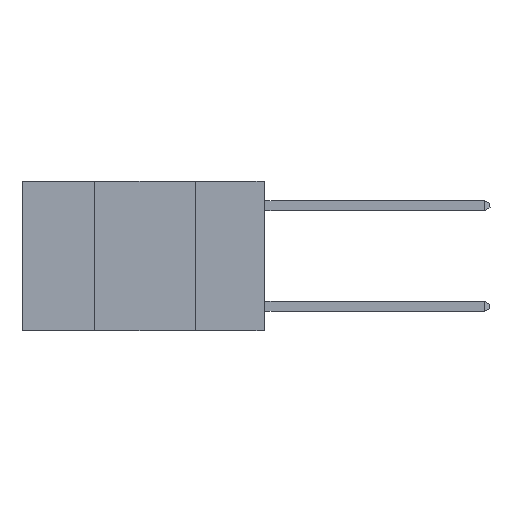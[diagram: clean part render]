
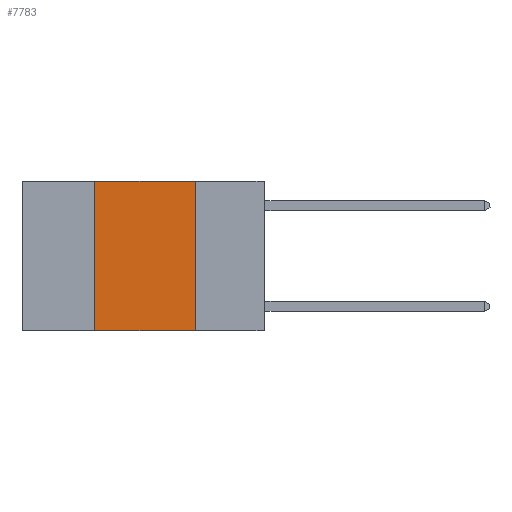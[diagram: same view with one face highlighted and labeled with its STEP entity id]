
A CAD part, left-side view. The second image highlights one B-rep face of the part: STEP entity #7783.
In plain terms, the highlighted planar face has unit normal (-1, 0, 0).
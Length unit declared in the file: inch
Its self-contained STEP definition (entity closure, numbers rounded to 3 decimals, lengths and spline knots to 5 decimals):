
#18 = CARTESIAN_POINT ( 'NONE',  ( 0., 0.6, 0. ) ) ;
#698 = DIRECTION ( 'NONE',  ( 0., -1., 0. ) ) ;
#1036 = PLANE ( 'NONE',  #8825 ) ;
#1455 = EDGE_CURVE ( 'NONE', #3841, #2883, #5703, .T. ) ;
#1847 = LINE ( 'NONE', #12381, #9710 ) ;
#2050 = DIRECTION ( 'NONE',  ( 0., 0., -1. ) ) ;
#2244 = ORIENTED_EDGE ( 'NONE', *, *, #5150, .T. ) ;
#2883 = VERTEX_POINT ( 'NONE', #4444 ) ;
#3067 = VERTEX_POINT ( 'NONE', #11845 ) ;
#3393 = ORIENTED_EDGE ( 'NONE', *, *, #1455, .F. ) ;
#3841 = VERTEX_POINT ( 'NONE', #10977 ) ;
#4159 = VECTOR ( 'NONE', #698, 39.37008 ) ;
#4444 = CARTESIAN_POINT ( 'NONE',  ( 0., 0.42, 0. ) ) ;
#4577 = ORIENTED_EDGE ( 'NONE', *, *, #6787, .F. ) ;
#4645 = ORIENTED_EDGE ( 'NONE', *, *, #4660, .F. ) ;
#4660 = EDGE_CURVE ( 'NONE', #6134, #3067, #10237, .T. ) ;
#4716 = EDGE_LOOP ( 'NONE', ( #4645, #4577, #3393, #2244 ) ) ;
#5006 = CARTESIAN_POINT ( 'NONE',  ( 0., 0.17, 0. ) ) ;
#5150 = EDGE_CURVE ( 'NONE', #3841, #3067, #9912, .T. ) ;
#5377 = VECTOR ( 'NONE', #8118, 39.37008 ) ;
#5703 = LINE ( 'NONE', #6126, #5377 ) ;
#5807 = CARTESIAN_POINT ( 'NONE',  ( 0., 0.6, -0.37 ) ) ;
#6039 = DIRECTION ( 'NONE',  ( 0., 0., -1. ) ) ;
#6126 = CARTESIAN_POINT ( 'NONE',  ( 0., 0.42, 0. ) ) ;
#6134 = VERTEX_POINT ( 'NONE', #11358 ) ;
#6787 = EDGE_CURVE ( 'NONE', #2883, #6134, #1847, .T. ) ;
#7285 = DIRECTION ( 'NONE',  ( 0., -1., 0. ) ) ;
#7783 = ADVANCED_FACE ( 'NONE', ( #8071 ), #1036, .F. ) ;
#8071 = FACE_OUTER_BOUND ( 'NONE', #4716, .T. ) ;
#8118 = DIRECTION ( 'NONE',  ( 0., 0., 1. ) ) ;
#8202 = DIRECTION ( 'NONE',  ( 1., 0., 0. ) ) ;
#8825 = AXIS2_PLACEMENT_3D ( 'NONE', #18, #8202, #2050 ) ;
#9710 = VECTOR ( 'NONE', #7285, 39.37008 ) ;
#9912 = LINE ( 'NONE', #5807, #4159 ) ;
#10237 = LINE ( 'NONE', #5006, #12641 ) ;
#10977 = CARTESIAN_POINT ( 'NONE',  ( 0., 0.42, -0.37 ) ) ;
#11358 = CARTESIAN_POINT ( 'NONE',  ( 0., 0.17, 0. ) ) ;
#11845 = CARTESIAN_POINT ( 'NONE',  ( 0., 0.17, -0.37 ) ) ;
#12381 = CARTESIAN_POINT ( 'NONE',  ( 0., 0.6, 0. ) ) ;
#12641 = VECTOR ( 'NONE', #6039, 39.37008 ) ;
